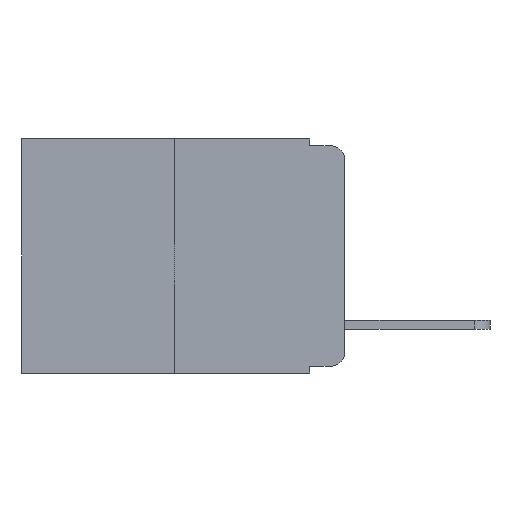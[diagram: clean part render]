
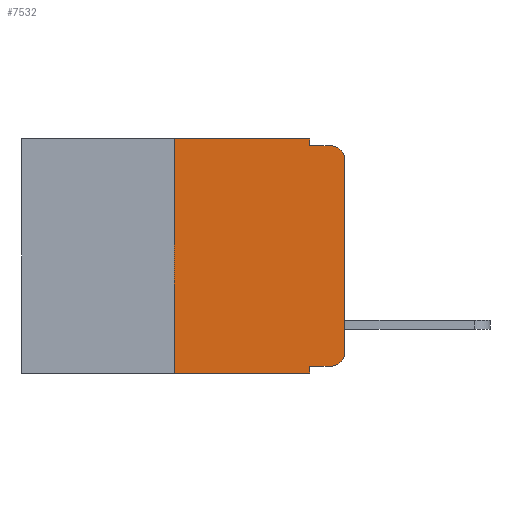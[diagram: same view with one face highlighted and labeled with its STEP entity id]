
A CAD part, left-side view. The second image highlights one B-rep face of the part: STEP entity #7532.
In plain terms, the highlighted planar face has unit normal (-1, 0, 0).
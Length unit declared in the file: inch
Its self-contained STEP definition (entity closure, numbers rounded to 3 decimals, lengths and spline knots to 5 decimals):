
#131 = AXIS2_PLACEMENT_3D ( 'NONE', #4987, #11120, #10080 ) ;
#161 = VECTOR ( 'NONE', #348, 39.37008 ) ;
#218 = CARTESIAN_POINT ( 'NONE',  ( 0., 0.473, 0. ) ) ;
#348 = DIRECTION ( 'NONE',  ( 0., 0., 1. ) ) ;
#354 = EDGE_CURVE ( 'NONE', #2607, #10069, #7865, .T. ) ;
#715 = CARTESIAN_POINT ( 'NONE',  ( 0., 0., -0.03 ) ) ;
#1044 = ORIENTED_EDGE ( 'NONE', *, *, #12223, .F. ) ;
#1491 = LINE ( 'NONE', #3175, #2292 ) ;
#1543 = CARTESIAN_POINT ( 'NONE',  ( 0., 0.25, -0.343 ) ) ;
#2292 = VECTOR ( 'NONE', #11227, 39.37008 ) ;
#2310 = VECTOR ( 'NONE', #11757, 39.37008 ) ;
#2436 = CARTESIAN_POINT ( 'NONE',  ( 0., 0.25, 0. ) ) ;
#2505 = DIRECTION ( 'NONE',  ( 0., 0., -1. ) ) ;
#2580 = EDGE_CURVE ( 'NONE', #3177, #5861, #6212, .T. ) ;
#2607 = VERTEX_POINT ( 'NONE', #10639 ) ;
#2610 = VECTOR ( 'NONE', #10795, 39.37008 ) ;
#2628 = CARTESIAN_POINT ( 'NONE',  ( 0., 0.473, -0.343 ) ) ;
#2633 = CARTESIAN_POINT ( 'NONE',  ( 0., 0.25, 0. ) ) ;
#2975 = CARTESIAN_POINT ( 'NONE',  ( 0., 0.051, -0.01 ) ) ;
#3175 = CARTESIAN_POINT ( 'NONE',  ( 0., 0., 0. ) ) ;
#3177 = VERTEX_POINT ( 'NONE', #1543 ) ;
#3439 = CARTESIAN_POINT ( 'NONE',  ( 0., 0.473, 0. ) ) ;
#3694 = EDGE_CURVE ( 'NONE', #10021, #7253, #8420, .T. ) ;
#3757 = ORIENTED_EDGE ( 'NONE', *, *, #7470, .T. ) ;
#3832 = VECTOR ( 'NONE', #8489, 39.37008 ) ;
#3933 = CARTESIAN_POINT ( 'NONE',  ( 0., 0.051, -0.01 ) ) ;
#4026 = DIRECTION ( 'NONE',  ( 0., -1., 0. ) ) ;
#4270 = LINE ( 'NONE', #10720, #11639 ) ;
#4791 = CARTESIAN_POINT ( 'NONE',  ( 0., 0.051, -0.333 ) ) ;
#4862 = EDGE_LOOP ( 'NONE', ( #10760, #12287, #9249, #11993, #10076, #8389, #3757, #1044, #8629, #10443 ) ) ;
#4987 = CARTESIAN_POINT ( 'NONE',  ( 0., 0.02, -0.313 ) ) ;
#5160 = CARTESIAN_POINT ( 'NONE',  ( 0., 0.051, 0. ) ) ;
#5282 = VERTEX_POINT ( 'NONE', #9378 ) ;
#5356 = CARTESIAN_POINT ( 'NONE',  ( 0., 0.02, -0.333 ) ) ;
#5543 = DIRECTION ( 'NONE',  ( 0., 0., -1. ) ) ;
#5861 = VERTEX_POINT ( 'NONE', #2633 ) ;
#6212 = LINE ( 'NONE', #2436, #161 ) ;
#6635 = LINE ( 'NONE', #2975, #10475 ) ;
#6748 = AXIS2_PLACEMENT_3D ( 'NONE', #218, #8525, #11945 ) ;
#7052 = FACE_OUTER_BOUND ( 'NONE', #4862, .T. ) ;
#7160 = VERTEX_POINT ( 'NONE', #8471 ) ;
#7253 = VERTEX_POINT ( 'NONE', #5356 ) ;
#7470 = EDGE_CURVE ( 'NONE', #3177, #10165, #12031, .T. ) ;
#7531 = EDGE_CURVE ( 'NONE', #5282, #11037, #1491, .T. ) ;
#7532 = ADVANCED_FACE ( 'NONE', ( #7052 ), #8323, .F. ) ;
#7537 = CIRCLE ( 'NONE', #8819, 0.02 ) ;
#7572 = CARTESIAN_POINT ( 'NONE',  ( 0., 0.02, -0.03 ) ) ;
#7660 = EDGE_CURVE ( 'NONE', #11037, #7160, #7537, .T. ) ;
#7865 = LINE ( 'NONE', #5160, #2310 ) ;
#8323 = PLANE ( 'NONE',  #6748 ) ;
#8389 = ORIENTED_EDGE ( 'NONE', *, *, #2580, .F. ) ;
#8420 = LINE ( 'NONE', #8876, #10019 ) ;
#8471 = CARTESIAN_POINT ( 'NONE',  ( 0., 0.02, -0.01 ) ) ;
#8489 = DIRECTION ( 'NONE',  ( 0., -1., 0. ) ) ;
#8525 = DIRECTION ( 'NONE',  ( 1., 0., 0. ) ) ;
#8629 = ORIENTED_EDGE ( 'NONE', *, *, #3694, .T. ) ;
#8805 = EDGE_CURVE ( 'NONE', #5861, #2607, #12793, .T. ) ;
#8819 = AXIS2_PLACEMENT_3D ( 'NONE', #7572, #11615, #2505 ) ;
#8876 = CARTESIAN_POINT ( 'NONE',  ( 0., 0.051, -0.333 ) ) ;
#9249 = ORIENTED_EDGE ( 'NONE', *, *, #10132, .F. ) ;
#9378 = CARTESIAN_POINT ( 'NONE',  ( 0., 0., -0.313 ) ) ;
#10019 = VECTOR ( 'NONE', #11874, 39.37008 ) ;
#10021 = VERTEX_POINT ( 'NONE', #4791 ) ;
#10069 = VERTEX_POINT ( 'NONE', #3933 ) ;
#10076 = ORIENTED_EDGE ( 'NONE', *, *, #8805, .F. ) ;
#10080 = DIRECTION ( 'NONE',  ( 0., 0., -1. ) ) ;
#10132 = EDGE_CURVE ( 'NONE', #10069, #7160, #6635, .T. ) ;
#10165 = VERTEX_POINT ( 'NONE', #12243 ) ;
#10271 = CIRCLE ( 'NONE', #131, 0.02 ) ;
#10443 = ORIENTED_EDGE ( 'NONE', *, *, #10983, .T. ) ;
#10475 = VECTOR ( 'NONE', #4026, 39.37008 ) ;
#10639 = CARTESIAN_POINT ( 'NONE',  ( 0., 0.051, 0. ) ) ;
#10720 = CARTESIAN_POINT ( 'NONE',  ( 0., 0.051, 0. ) ) ;
#10760 = ORIENTED_EDGE ( 'NONE', *, *, #7531, .T. ) ;
#10795 = DIRECTION ( 'NONE',  ( 0., -1., 0. ) ) ;
#10983 = EDGE_CURVE ( 'NONE', #7253, #5282, #10271, .T. ) ;
#11037 = VERTEX_POINT ( 'NONE', #715 ) ;
#11120 = DIRECTION ( 'NONE',  ( -1., 0., 0. ) ) ;
#11227 = DIRECTION ( 'NONE',  ( 0., 0., 1. ) ) ;
#11615 = DIRECTION ( 'NONE',  ( -1., 0., 0. ) ) ;
#11639 = VECTOR ( 'NONE', #5543, 39.37008 ) ;
#11757 = DIRECTION ( 'NONE',  ( 0., 0., -1. ) ) ;
#11874 = DIRECTION ( 'NONE',  ( 0., -1., 0. ) ) ;
#11945 = DIRECTION ( 'NONE',  ( 0., 0., -1. ) ) ;
#11993 = ORIENTED_EDGE ( 'NONE', *, *, #354, .F. ) ;
#12031 = LINE ( 'NONE', #2628, #2610 ) ;
#12223 = EDGE_CURVE ( 'NONE', #10021, #10165, #4270, .T. ) ;
#12243 = CARTESIAN_POINT ( 'NONE',  ( 0., 0.051, -0.343 ) ) ;
#12287 = ORIENTED_EDGE ( 'NONE', *, *, #7660, .T. ) ;
#12793 = LINE ( 'NONE', #3439, #3832 ) ;
